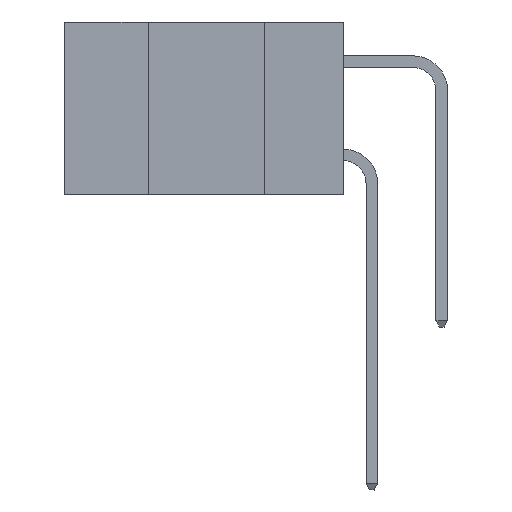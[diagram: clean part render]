
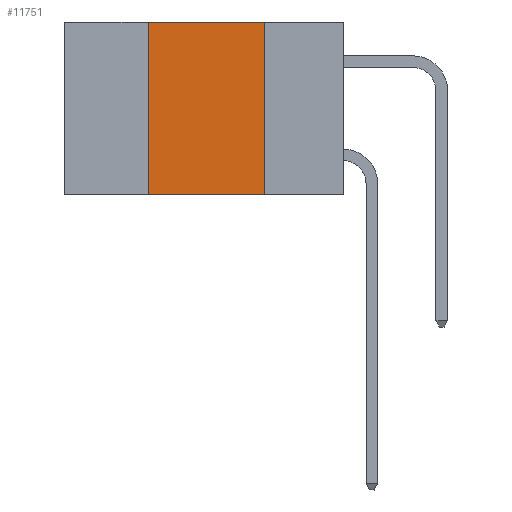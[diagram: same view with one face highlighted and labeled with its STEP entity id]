
A CAD part, left-side view. The second image highlights one B-rep face of the part: STEP entity #11751.
In plain terms, the highlighted planar face has unit normal (-1, 0, 0).
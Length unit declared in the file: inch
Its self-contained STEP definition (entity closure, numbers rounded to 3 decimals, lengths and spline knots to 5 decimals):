
#126 = VECTOR ( 'NONE', #9312, 39.37008 ) ;
#1656 = LINE ( 'NONE', #10303, #6655 ) ;
#1902 = ORIENTED_EDGE ( 'NONE', *, *, #14052, .F. ) ;
#2210 = DIRECTION ( 'NONE',  ( 0., -1., 0. ) ) ;
#2374 = LINE ( 'NONE', #9796, #9870 ) ;
#3290 = ORIENTED_EDGE ( 'NONE', *, *, #6025, .F. ) ;
#3547 = DIRECTION ( 'NONE',  ( 1., 0., 0. ) ) ;
#3799 = VECTOR ( 'NONE', #7757, 39.37008 ) ;
#3888 = CARTESIAN_POINT ( 'NONE',  ( 0., 0.42, -0.37 ) ) ;
#4528 = FACE_OUTER_BOUND ( 'NONE', #10076, .T. ) ;
#5808 = CARTESIAN_POINT ( 'NONE',  ( 0., 0.17, -0.37 ) ) ;
#6012 = EDGE_CURVE ( 'NONE', #6701, #10173, #1656, .T. ) ;
#6025 = EDGE_CURVE ( 'NONE', #6701, #14469, #7933, .T. ) ;
#6442 = VERTEX_POINT ( 'NONE', #15257 ) ;
#6625 = DIRECTION ( 'NONE',  ( 0., -1., 0. ) ) ;
#6655 = VECTOR ( 'NONE', #6625, 39.37008 ) ;
#6701 = VERTEX_POINT ( 'NONE', #3888 ) ;
#7757 = DIRECTION ( 'NONE',  ( 0., 0., -1. ) ) ;
#7844 = CARTESIAN_POINT ( 'NONE',  ( 0., 0.17, -0.37 ) ) ;
#7933 = LINE ( 'NONE', #14142, #126 ) ;
#8834 = ORIENTED_EDGE ( 'NONE', *, *, #6012, .T. ) ;
#9312 = DIRECTION ( 'NONE',  ( 0., 0., 1. ) ) ;
#9498 = PLANE ( 'NONE',  #14259 ) ;
#9796 = CARTESIAN_POINT ( 'NONE',  ( 0., 0.6, 0. ) ) ;
#9870 = VECTOR ( 'NONE', #2210, 39.37008 ) ;
#9997 = EDGE_CURVE ( 'NONE', #6442, #10173, #13442, .T. ) ;
#10076 = EDGE_LOOP ( 'NONE', ( #10236, #1902, #3290, #8834 ) ) ;
#10173 = VERTEX_POINT ( 'NONE', #5808 ) ;
#10236 = ORIENTED_EDGE ( 'NONE', *, *, #9997, .F. ) ;
#10303 = CARTESIAN_POINT ( 'NONE',  ( 0., 0.6, -0.37 ) ) ;
#11751 = ADVANCED_FACE ( 'NONE', ( #4528 ), #9498, .F. ) ;
#12356 = DIRECTION ( 'NONE',  ( 0., 0., -1. ) ) ;
#13258 = CARTESIAN_POINT ( 'NONE',  ( 0., 0.6, 0. ) ) ;
#13442 = LINE ( 'NONE', #7844, #3799 ) ;
#14052 = EDGE_CURVE ( 'NONE', #14469, #6442, #2374, .T. ) ;
#14142 = CARTESIAN_POINT ( 'NONE',  ( 0., 0.42, -0.37 ) ) ;
#14259 = AXIS2_PLACEMENT_3D ( 'NONE', #13258, #3547, #12356 ) ;
#14266 = CARTESIAN_POINT ( 'NONE',  ( 0., 0.42, 0. ) ) ;
#14469 = VERTEX_POINT ( 'NONE', #14266 ) ;
#15257 = CARTESIAN_POINT ( 'NONE',  ( 0., 0.17, 0. ) ) ;
